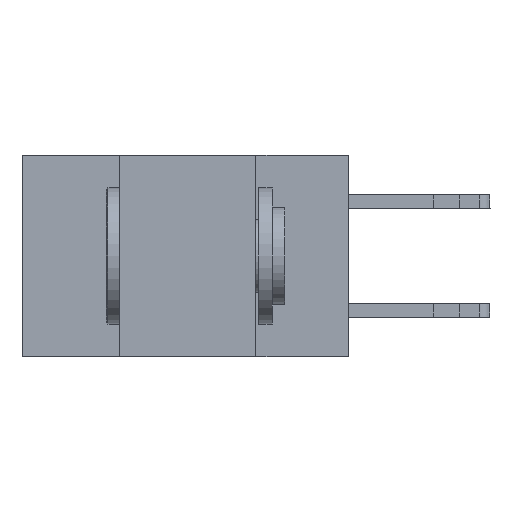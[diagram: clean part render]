
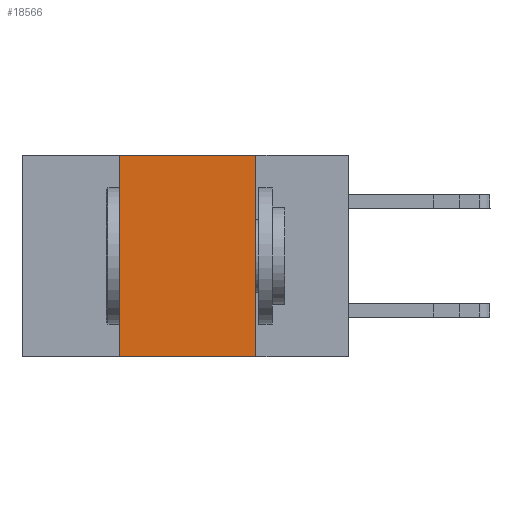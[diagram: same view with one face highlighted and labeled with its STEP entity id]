
A CAD part, left-side view. The second image highlights one B-rep face of the part: STEP entity #18566.
In plain terms, the highlighted planar face has unit normal (-1, 0, 0).
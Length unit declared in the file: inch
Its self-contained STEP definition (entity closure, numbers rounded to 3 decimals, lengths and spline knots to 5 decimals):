
#168 = CARTESIAN_POINT ( 'NONE',  ( 0., 0.42, -0.37 ) ) ;
#1276 = EDGE_CURVE ( 'NONE', #21283, #11105, #9492, .T. ) ;
#1841 = EDGE_LOOP ( 'NONE', ( #13174, #14568, #18551, #11733 ) ) ;
#2792 = CARTESIAN_POINT ( 'NONE',  ( 0., 0.17, -0.37 ) ) ;
#3054 = VERTEX_POINT ( 'NONE', #19766 ) ;
#3143 = CARTESIAN_POINT ( 'NONE',  ( 0., 0.6, 0. ) ) ;
#3295 = VECTOR ( 'NONE', #4473, 39.37008 ) ;
#4402 = EDGE_CURVE ( 'NONE', #3054, #21283, #21240, .T. ) ;
#4473 = DIRECTION ( 'NONE',  ( 0., 0., -1. ) ) ;
#4774 = EDGE_CURVE ( 'NONE', #8224, #3054, #15493, .T. ) ;
#7015 = DIRECTION ( 'NONE',  ( 0., 0., 1. ) ) ;
#8224 = VERTEX_POINT ( 'NONE', #16507 ) ;
#8762 = LINE ( 'NONE', #10896, #20869 ) ;
#8812 = VECTOR ( 'NONE', #7015, 39.37008 ) ;
#8882 = DIRECTION ( 'NONE',  ( 0., -1., 0. ) ) ;
#9492 = LINE ( 'NONE', #2792, #3295 ) ;
#10831 = DIRECTION ( 'NONE',  ( 0., -1., 0. ) ) ;
#10896 = CARTESIAN_POINT ( 'NONE',  ( 0., 0.6, -0.37 ) ) ;
#11105 = VERTEX_POINT ( 'NONE', #19684 ) ;
#11733 = ORIENTED_EDGE ( 'NONE', *, *, #13130, .T. ) ;
#11838 = DIRECTION ( 'NONE',  ( 1., 0., 0. ) ) ;
#12623 = CARTESIAN_POINT ( 'NONE',  ( 0., 0.6, 0. ) ) ;
#13130 = EDGE_CURVE ( 'NONE', #8224, #11105, #8762, .T. ) ;
#13174 = ORIENTED_EDGE ( 'NONE', *, *, #1276, .F. ) ;
#14568 = ORIENTED_EDGE ( 'NONE', *, *, #4402, .F. ) ;
#15493 = LINE ( 'NONE', #168, #8812 ) ;
#16507 = CARTESIAN_POINT ( 'NONE',  ( 0., 0.42, -0.37 ) ) ;
#18462 = PLANE ( 'NONE',  #21259 ) ;
#18551 = ORIENTED_EDGE ( 'NONE', *, *, #4774, .F. ) ;
#18566 = ADVANCED_FACE ( 'NONE', ( #20125 ), #18462, .F. ) ;
#18674 = DIRECTION ( 'NONE',  ( 0., 0., -1. ) ) ;
#19684 = CARTESIAN_POINT ( 'NONE',  ( 0., 0.17, -0.37 ) ) ;
#19766 = CARTESIAN_POINT ( 'NONE',  ( 0., 0.42, 0. ) ) ;
#19939 = CARTESIAN_POINT ( 'NONE',  ( 0., 0.17, 0. ) ) ;
#20125 = FACE_OUTER_BOUND ( 'NONE', #1841, .T. ) ;
#20590 = VECTOR ( 'NONE', #10831, 39.37008 ) ;
#20869 = VECTOR ( 'NONE', #8882, 39.37008 ) ;
#21240 = LINE ( 'NONE', #12623, #20590 ) ;
#21259 = AXIS2_PLACEMENT_3D ( 'NONE', #3143, #11838, #18674 ) ;
#21283 = VERTEX_POINT ( 'NONE', #19939 ) ;
